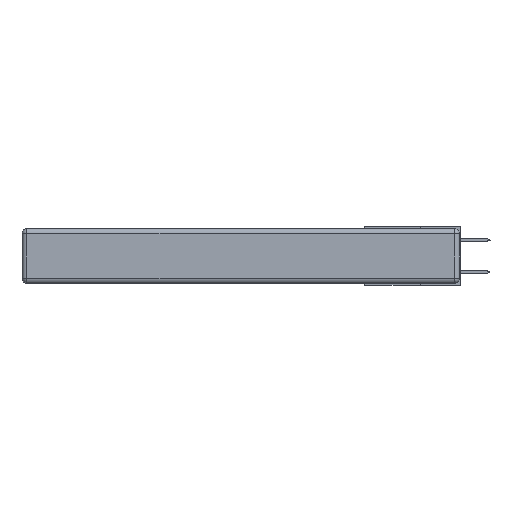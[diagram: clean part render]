
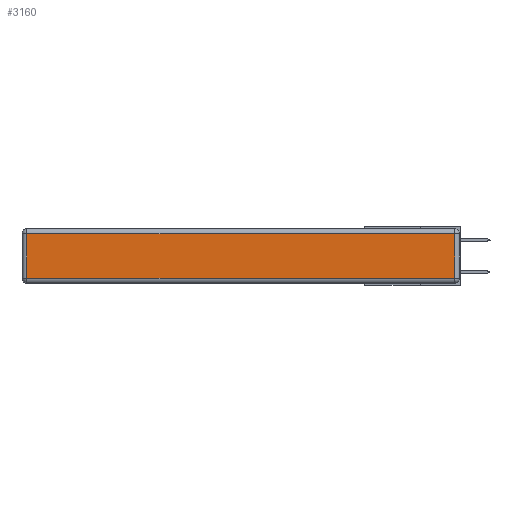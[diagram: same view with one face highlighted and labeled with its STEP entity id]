
A CAD part, left-side view. The second image highlights one B-rep face of the part: STEP entity #3160.
In plain terms, the highlighted planar face has unit normal (-1, 0, 0).
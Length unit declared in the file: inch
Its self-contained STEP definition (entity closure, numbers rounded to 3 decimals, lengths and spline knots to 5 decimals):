
#265 = ORIENTED_EDGE ( 'NONE', *, *, #11968, .T. ) ;
#297 = CARTESIAN_POINT ( 'NONE',  ( 0., 0.03, -0.03 ) ) ;
#409 = VERTEX_POINT ( 'NONE', #8306 ) ;
#770 = VECTOR ( 'NONE', #5095, 39.37008 ) ;
#2181 = VECTOR ( 'NONE', #11212, 39.37008 ) ;
#2316 = EDGE_LOOP ( 'NONE', ( #8538, #6496, #10069, #265 ) ) ;
#2505 = VECTOR ( 'NONE', #7759, 39.37008 ) ;
#2691 = FACE_OUTER_BOUND ( 'NONE', #2316, .T. ) ;
#2930 = LINE ( 'NONE', #4274, #2181 ) ;
#3067 = CARTESIAN_POINT ( 'NONE',  ( 0., 2.72, -0.03 ) ) ;
#3160 = ADVANCED_FACE ( 'NONE', ( #2691 ), #3862, .T. ) ;
#3285 = CARTESIAN_POINT ( 'NONE',  ( 0., 2.72, -0.313 ) ) ;
#3394 = LINE ( 'NONE', #4053, #770 ) ;
#3862 = PLANE ( 'NONE',  #8687 ) ;
#4053 = CARTESIAN_POINT ( 'NONE',  ( 0., 0.03, -0.343 ) ) ;
#4217 = VERTEX_POINT ( 'NONE', #3067 ) ;
#4274 = CARTESIAN_POINT ( 'NONE',  ( 0., 2.75, -0.03 ) ) ;
#4870 = DIRECTION ( 'NONE',  ( -1., 0., 0. ) ) ;
#5095 = DIRECTION ( 'NONE',  ( 0., 0., 1. ) ) ;
#5661 = CARTESIAN_POINT ( 'NONE',  ( 0., 2.72, -0.343 ) ) ;
#5818 = CARTESIAN_POINT ( 'NONE',  ( 0., 0., -0.343 ) ) ;
#6496 = ORIENTED_EDGE ( 'NONE', *, *, #7567, .T. ) ;
#6983 = EDGE_CURVE ( 'NONE', #12326, #4217, #2930, .T. ) ;
#7142 = DIRECTION ( 'NONE',  ( 0., -1., 0. ) ) ;
#7193 = CARTESIAN_POINT ( 'NONE',  ( 0., 0., -0.313 ) ) ;
#7500 = EDGE_CURVE ( 'NONE', #11503, #409, #10263, .T. ) ;
#7567 = EDGE_CURVE ( 'NONE', #409, #12326, #3394, .T. ) ;
#7666 = DIRECTION ( 'NONE',  ( 0., 0., 1. ) ) ;
#7759 = DIRECTION ( 'NONE',  ( 0., 0., -1. ) ) ;
#8306 = CARTESIAN_POINT ( 'NONE',  ( 0., 0.03, -0.313 ) ) ;
#8538 = ORIENTED_EDGE ( 'NONE', *, *, #7500, .T. ) ;
#8687 = AXIS2_PLACEMENT_3D ( 'NONE', #5818, #4870, #7666 ) ;
#9959 = LINE ( 'NONE', #5661, #2505 ) ;
#10069 = ORIENTED_EDGE ( 'NONE', *, *, #6983, .T. ) ;
#10263 = LINE ( 'NONE', #7193, #11334 ) ;
#11212 = DIRECTION ( 'NONE',  ( 0., 1., 0. ) ) ;
#11334 = VECTOR ( 'NONE', #7142, 39.37008 ) ;
#11503 = VERTEX_POINT ( 'NONE', #3285 ) ;
#11968 = EDGE_CURVE ( 'NONE', #4217, #11503, #9959, .T. ) ;
#12326 = VERTEX_POINT ( 'NONE', #297 ) ;
